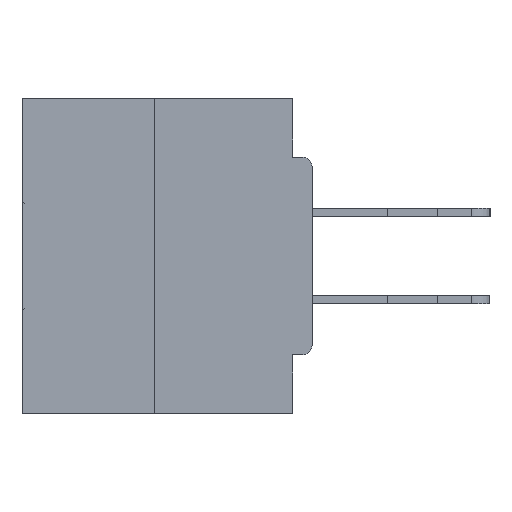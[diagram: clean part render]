
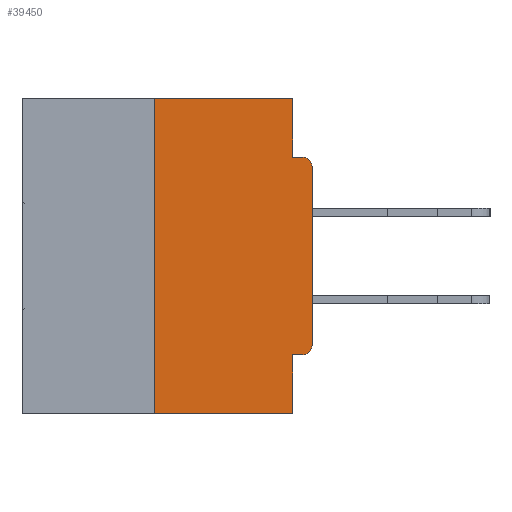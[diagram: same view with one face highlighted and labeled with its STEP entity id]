
A CAD part, left-side view. The second image highlights one B-rep face of the part: STEP entity #39450.
In plain terms, the highlighted planar face has unit normal (-1, 0, 0).
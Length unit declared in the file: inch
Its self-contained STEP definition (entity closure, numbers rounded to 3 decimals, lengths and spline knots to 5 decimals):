
#24 = AXIS2_PLACEMENT_3D ( 'NONE', #20155, #35871, #33107 ) ;
#38 = CARTESIAN_POINT ( 'NONE',  ( 0., 0., 0. ) ) ;
#852 = VECTOR ( 'NONE', #41447, 39.37008 ) ;
#1811 = CARTESIAN_POINT ( 'NONE',  ( 0., 0.015, -0.0935 ) ) ;
#4590 = VECTOR ( 'NONE', #37856, 39.37008 ) ;
#4649 = CARTESIAN_POINT ( 'NONE',  ( 0., 0.25, 0. ) ) ;
#5246 = ORIENTED_EDGE ( 'NONE', *, *, #37339, .F. ) ;
#5554 = EDGE_CURVE ( 'NONE', #29200, #11923, #9250, .T. ) ;
#5652 = AXIS2_PLACEMENT_3D ( 'NONE', #40885, #41011, #21622 ) ;
#5896 = FACE_OUTER_BOUND ( 'NONE', #35239, .T. ) ;
#6063 = VERTEX_POINT ( 'NONE', #10382 ) ;
#6606 = CARTESIAN_POINT ( 'NONE',  ( 0., 0.031, -0.0935 ) ) ;
#7060 = EDGE_CURVE ( 'NONE', #25362, #26168, #27344, .T. ) ;
#7540 = VERTEX_POINT ( 'NONE', #40310 ) ;
#7563 = DIRECTION ( 'NONE',  ( 0., -1., 0. ) ) ;
#7732 = EDGE_CURVE ( 'NONE', #24152, #30917, #8630, .T. ) ;
#8381 = DIRECTION ( 'NONE',  ( 0., 0., -1. ) ) ;
#8630 = LINE ( 'NONE', #15383, #4590 ) ;
#8906 = DIRECTION ( 'NONE',  ( 0., 0., -1. ) ) ;
#9250 = LINE ( 'NONE', #38, #11789 ) ;
#9444 = LINE ( 'NONE', #25143, #852 ) ;
#10116 = ORIENTED_EDGE ( 'NONE', *, *, #37952, .F. ) ;
#10382 = CARTESIAN_POINT ( 'NONE',  ( 0., 0.031, 0. ) ) ;
#10621 = CARTESIAN_POINT ( 'NONE',  ( 0., 0., -0.4065 ) ) ;
#11789 = VECTOR ( 'NONE', #37551, 39.37008 ) ;
#11923 = VERTEX_POINT ( 'NONE', #24156 ) ;
#12156 = EDGE_CURVE ( 'NONE', #7540, #29200, #33481, .T. ) ;
#12200 = CARTESIAN_POINT ( 'NONE',  ( 0., 0.46, 0. ) ) ;
#12592 = CIRCLE ( 'NONE', #5652, 0.015 ) ;
#13822 = PLANE ( 'NONE',  #24 ) ;
#14120 = DIRECTION ( 'NONE',  ( 0., 1., 0. ) ) ;
#14415 = DIRECTION ( 'NONE',  ( -1., 0., 0. ) ) ;
#14440 = AXIS2_PLACEMENT_3D ( 'NONE', #14983, #14415, #8381 ) ;
#14983 = CARTESIAN_POINT ( 'NONE',  ( 0., 0.015, -0.3915 ) ) ;
#15022 = EDGE_CURVE ( 'NONE', #11923, #31963, #12592, .T. ) ;
#15383 = CARTESIAN_POINT ( 'NONE',  ( 0., 0.031, -0.5 ) ) ;
#17756 = ORIENTED_EDGE ( 'NONE', *, *, #15022, .T. ) ;
#18485 = EDGE_CURVE ( 'NONE', #7540, #24152, #37453, .T. ) ;
#18840 = VECTOR ( 'NONE', #14120, 39.37008 ) ;
#18954 = LINE ( 'NONE', #22100, #35065 ) ;
#19162 = LINE ( 'NONE', #26862, #31781 ) ;
#19531 = ORIENTED_EDGE ( 'NONE', *, *, #5554, .T. ) ;
#19603 = VECTOR ( 'NONE', #34709, 39.37008 ) ;
#19680 = CARTESIAN_POINT ( 'NONE',  ( 0., 0.031, -0.4065 ) ) ;
#20155 = CARTESIAN_POINT ( 'NONE',  ( 0., 0.46, 0. ) ) ;
#21573 = VERTEX_POINT ( 'NONE', #6606 ) ;
#21622 = DIRECTION ( 'NONE',  ( 0., 0., -1. ) ) ;
#22100 = CARTESIAN_POINT ( 'NONE',  ( 0., 0.031, 0. ) ) ;
#22511 = ORIENTED_EDGE ( 'NONE', *, *, #7732, .F. ) ;
#23837 = ORIENTED_EDGE ( 'NONE', *, *, #7060, .F. ) ;
#24152 = VERTEX_POINT ( 'NONE', #19680 ) ;
#24156 = CARTESIAN_POINT ( 'NONE',  ( 0., 0., -0.1085 ) ) ;
#24547 = CARTESIAN_POINT ( 'NONE',  ( 0., 0., -0.3915 ) ) ;
#24677 = LINE ( 'NONE', #12200, #19603 ) ;
#25143 = CARTESIAN_POINT ( 'NONE',  ( 0., 0.46, -0.5 ) ) ;
#25362 = VERTEX_POINT ( 'NONE', #38879 ) ;
#26168 = VERTEX_POINT ( 'NONE', #37904 ) ;
#26862 = CARTESIAN_POINT ( 'NONE',  ( 0., 0., -0.0935 ) ) ;
#27344 = LINE ( 'NONE', #4649, #29298 ) ;
#28834 = ORIENTED_EDGE ( 'NONE', *, *, #34403, .T. ) ;
#29200 = VERTEX_POINT ( 'NONE', #24547 ) ;
#29298 = VECTOR ( 'NONE', #33623, 39.37008 ) ;
#30917 = VERTEX_POINT ( 'NONE', #40211 ) ;
#31781 = VECTOR ( 'NONE', #7563, 39.37008 ) ;
#31963 = VERTEX_POINT ( 'NONE', #1811 ) ;
#33107 = DIRECTION ( 'NONE',  ( 0., 0., -1. ) ) ;
#33346 = ORIENTED_EDGE ( 'NONE', *, *, #12156, .T. ) ;
#33481 = CIRCLE ( 'NONE', #14440, 0.015 ) ;
#33623 = DIRECTION ( 'NONE',  ( 0., 0., 1. ) ) ;
#34403 = EDGE_CURVE ( 'NONE', #25362, #30917, #9444, .T. ) ;
#34709 = DIRECTION ( 'NONE',  ( 0., -1., 0. ) ) ;
#35065 = VECTOR ( 'NONE', #8906, 39.37008 ) ;
#35239 = EDGE_LOOP ( 'NONE', ( #10116, #23837, #28834, #22511, #39145, #33346, #19531, #17756, #5246, #40159 ) ) ;
#35871 = DIRECTION ( 'NONE',  ( 1., 0., 0. ) ) ;
#37339 = EDGE_CURVE ( 'NONE', #21573, #31963, #19162, .T. ) ;
#37453 = LINE ( 'NONE', #10621, #18840 ) ;
#37551 = DIRECTION ( 'NONE',  ( 0., 0., 1. ) ) ;
#37856 = DIRECTION ( 'NONE',  ( 0., 0., -1. ) ) ;
#37904 = CARTESIAN_POINT ( 'NONE',  ( 0., 0.25, 0. ) ) ;
#37952 = EDGE_CURVE ( 'NONE', #26168, #6063, #24677, .T. ) ;
#38879 = CARTESIAN_POINT ( 'NONE',  ( 0., 0.25, -0.5 ) ) ;
#38977 = EDGE_CURVE ( 'NONE', #6063, #21573, #18954, .T. ) ;
#39145 = ORIENTED_EDGE ( 'NONE', *, *, #18485, .F. ) ;
#39450 = ADVANCED_FACE ( 'NONE', ( #5896 ), #13822, .F. ) ;
#40159 = ORIENTED_EDGE ( 'NONE', *, *, #38977, .F. ) ;
#40211 = CARTESIAN_POINT ( 'NONE',  ( 0., 0.031, -0.5 ) ) ;
#40310 = CARTESIAN_POINT ( 'NONE',  ( 0., 0.015, -0.4065 ) ) ;
#40885 = CARTESIAN_POINT ( 'NONE',  ( 0., 0.015, -0.1085 ) ) ;
#41011 = DIRECTION ( 'NONE',  ( -1., 0., 0. ) ) ;
#41447 = DIRECTION ( 'NONE',  ( 0., -1., 0. ) ) ;
